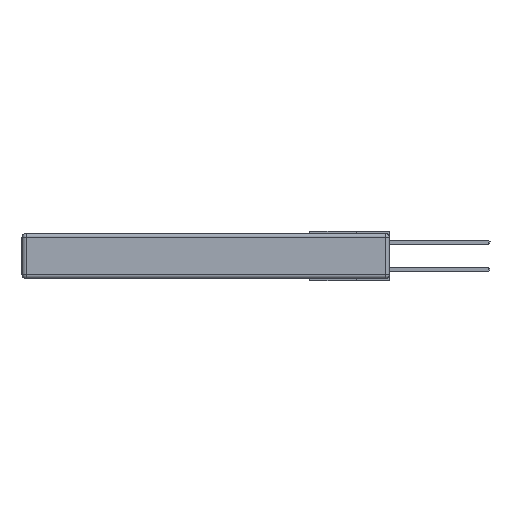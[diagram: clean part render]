
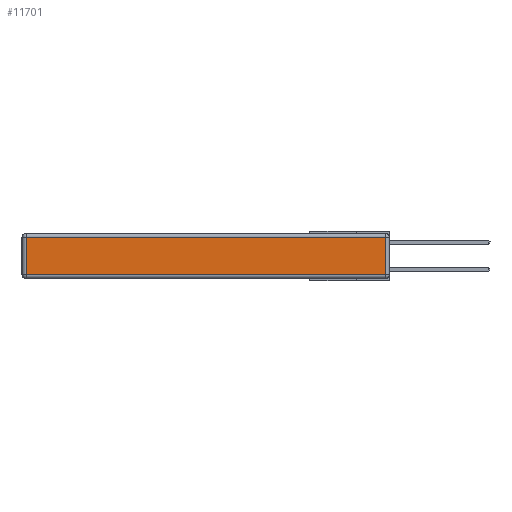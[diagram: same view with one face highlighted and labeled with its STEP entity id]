
A CAD part, left-side view. The second image highlights one B-rep face of the part: STEP entity #11701.
In plain terms, the highlighted planar face has unit normal (-1, 0, 0).
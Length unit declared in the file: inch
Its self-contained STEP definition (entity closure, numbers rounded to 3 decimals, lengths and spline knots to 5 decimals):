
#49 = LINE ( 'NONE', #12411, #12897 ) ;
#1328 = ORIENTED_EDGE ( 'NONE', *, *, #24827, .T. ) ;
#2449 = AXIS2_PLACEMENT_3D ( 'NONE', #19445, #11390, #25197 ) ;
#4469 = DIRECTION ( 'NONE',  ( 0., 1., 0. ) ) ;
#4606 = ORIENTED_EDGE ( 'NONE', *, *, #5014, .T. ) ;
#5014 = EDGE_CURVE ( 'NONE', #12418, #14491, #10077, .T. ) ;
#5072 = EDGE_CURVE ( 'NONE', #15618, #5858, #14672, .T. ) ;
#5858 = VERTEX_POINT ( 'NONE', #9563 ) ;
#6425 = DIRECTION ( 'NONE',  ( 0., 0., 1. ) ) ;
#6688 = DIRECTION ( 'NONE',  ( 0., 0., -1. ) ) ;
#8273 = CARTESIAN_POINT ( 'NONE',  ( 0., 0.03, -0.03 ) ) ;
#8325 = CARTESIAN_POINT ( 'NONE',  ( 0., 0.03, -0.343 ) ) ;
#9563 = CARTESIAN_POINT ( 'NONE',  ( 0., 2.72, -0.313 ) ) ;
#10077 = LINE ( 'NONE', #8325, #10668 ) ;
#10668 = VECTOR ( 'NONE', #6425, 39.37008 ) ;
#11030 = VECTOR ( 'NONE', #11281, 39.37008 ) ;
#11281 = DIRECTION ( 'NONE',  ( 0., -1., 0. ) ) ;
#11390 = DIRECTION ( 'NONE',  ( -1., 0., 0. ) ) ;
#11399 = ORIENTED_EDGE ( 'NONE', *, *, #5072, .T. ) ;
#11701 = ADVANCED_FACE ( 'NONE', ( #14647 ), #21318, .T. ) ;
#12264 = LINE ( 'NONE', #19157, #11030 ) ;
#12411 = CARTESIAN_POINT ( 'NONE',  ( 0., 2.75, -0.03 ) ) ;
#12418 = VERTEX_POINT ( 'NONE', #14333 ) ;
#12897 = VECTOR ( 'NONE', #4469, 39.37008 ) ;
#14333 = CARTESIAN_POINT ( 'NONE',  ( 0., 0.03, -0.313 ) ) ;
#14491 = VERTEX_POINT ( 'NONE', #8273 ) ;
#14647 = FACE_OUTER_BOUND ( 'NONE', #14856, .T. ) ;
#14672 = LINE ( 'NONE', #20554, #17808 ) ;
#14856 = EDGE_LOOP ( 'NONE', ( #15873, #4606, #1328, #11399 ) ) ;
#15618 = VERTEX_POINT ( 'NONE', #24949 ) ;
#15873 = ORIENTED_EDGE ( 'NONE', *, *, #16283, .T. ) ;
#16283 = EDGE_CURVE ( 'NONE', #5858, #12418, #12264, .T. ) ;
#17808 = VECTOR ( 'NONE', #6688, 39.37008 ) ;
#19157 = CARTESIAN_POINT ( 'NONE',  ( 0., 0., -0.313 ) ) ;
#19445 = CARTESIAN_POINT ( 'NONE',  ( 0., 0., -0.343 ) ) ;
#20554 = CARTESIAN_POINT ( 'NONE',  ( 0., 2.72, -0.343 ) ) ;
#21318 = PLANE ( 'NONE',  #2449 ) ;
#24827 = EDGE_CURVE ( 'NONE', #14491, #15618, #49, .T. ) ;
#24949 = CARTESIAN_POINT ( 'NONE',  ( 0., 2.72, -0.03 ) ) ;
#25197 = DIRECTION ( 'NONE',  ( 0., 0., 1. ) ) ;
